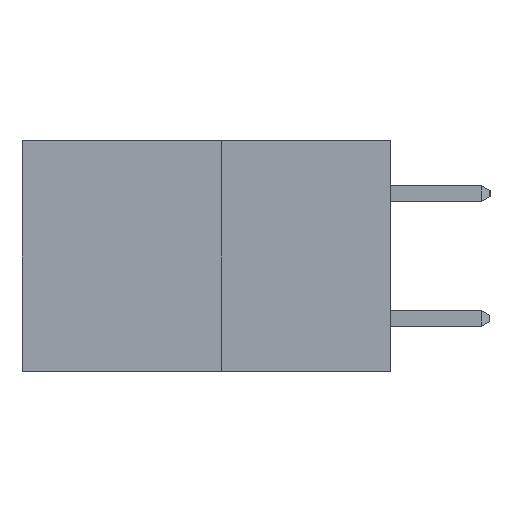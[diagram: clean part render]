
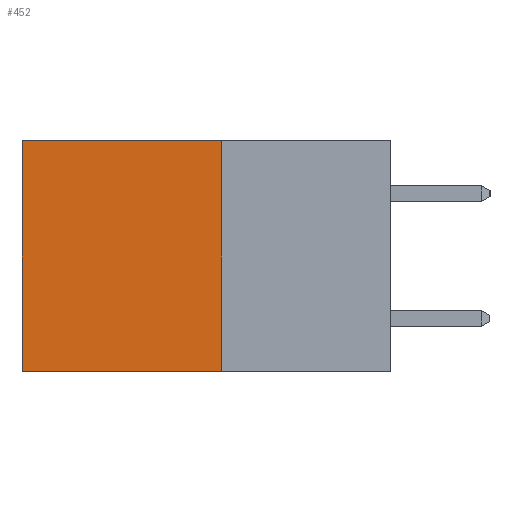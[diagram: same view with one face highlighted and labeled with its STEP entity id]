
A CAD part, left-side view. The second image highlights one B-rep face of the part: STEP entity #452.
In plain terms, the highlighted planar face has unit normal (-1, 0, 0).
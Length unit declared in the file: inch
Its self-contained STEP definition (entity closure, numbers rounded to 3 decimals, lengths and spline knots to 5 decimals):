
#408 = ORIENTED_EDGE ( 'NONE', *, *, #8867, .F. ) ;
#452 = ADVANCED_FACE ( 'NONE', ( #4900 ), #4227, .F. ) ;
#484 = EDGE_CURVE ( 'NONE', #5324, #876, #8428, .T. ) ;
#602 = CARTESIAN_POINT ( 'NONE',  ( 0.277, 0.27, -0.37 ) ) ;
#876 = VERTEX_POINT ( 'NONE', #3159 ) ;
#1365 = ORIENTED_EDGE ( 'NONE', *, *, #484, .T. ) ;
#1741 = LINE ( 'NONE', #7117, #4344 ) ;
#1818 = VECTOR ( 'NONE', #8459, 39.37008 ) ;
#2048 = CARTESIAN_POINT ( 'NONE',  ( 0.277, 0.27, 0. ) ) ;
#2749 = CARTESIAN_POINT ( 'NONE',  ( 0.277, 0.59, -0.37 ) ) ;
#2950 = ORIENTED_EDGE ( 'NONE', *, *, #9216, .F. ) ;
#3159 = CARTESIAN_POINT ( 'NONE',  ( 0.277, 0.59, -0.37 ) ) ;
#3672 = DIRECTION ( 'NONE',  ( 0., 0., -1. ) ) ;
#3868 = LINE ( 'NONE', #602, #7657 ) ;
#4227 = PLANE ( 'NONE',  #6699 ) ;
#4344 = VECTOR ( 'NONE', #6665, 39.37008 ) ;
#4402 = LINE ( 'NONE', #8374, #1818 ) ;
#4900 = FACE_OUTER_BOUND ( 'NONE', #8016, .T. ) ;
#5074 = CARTESIAN_POINT ( 'NONE',  ( 0.277, 0.27, -0.37 ) ) ;
#5324 = VERTEX_POINT ( 'NONE', #5848 ) ;
#5383 = CARTESIAN_POINT ( 'NONE',  ( 0.277, 0.27, -0.37 ) ) ;
#5848 = CARTESIAN_POINT ( 'NONE',  ( 0.277, 0.59, 0. ) ) ;
#5937 = ORIENTED_EDGE ( 'NONE', *, *, #6029, .T. ) ;
#6029 = EDGE_CURVE ( 'NONE', #9110, #5324, #1741, .T. ) ;
#6200 = VECTOR ( 'NONE', #3672, 39.37008 ) ;
#6458 = DIRECTION ( 'NONE',  ( 0., 1., 0. ) ) ;
#6665 = DIRECTION ( 'NONE',  ( 0., 1., 0. ) ) ;
#6699 = AXIS2_PLACEMENT_3D ( 'NONE', #5383, #7045, #7085 ) ;
#7045 = DIRECTION ( 'NONE',  ( 1., 0., 0. ) ) ;
#7085 = DIRECTION ( 'NONE',  ( 0., 0., -1. ) ) ;
#7117 = CARTESIAN_POINT ( 'NONE',  ( 0.277, 0.27, 0. ) ) ;
#7552 = VERTEX_POINT ( 'NONE', #5074 ) ;
#7657 = VECTOR ( 'NONE', #6458, 39.37008 ) ;
#8016 = EDGE_LOOP ( 'NONE', ( #1365, #2950, #408, #5937 ) ) ;
#8374 = CARTESIAN_POINT ( 'NONE',  ( 0.277, 0.27, -0.37 ) ) ;
#8428 = LINE ( 'NONE', #2749, #6200 ) ;
#8459 = DIRECTION ( 'NONE',  ( 0., 0., -1. ) ) ;
#8867 = EDGE_CURVE ( 'NONE', #9110, #7552, #4402, .T. ) ;
#9110 = VERTEX_POINT ( 'NONE', #2048 ) ;
#9216 = EDGE_CURVE ( 'NONE', #7552, #876, #3868, .T. ) ;
